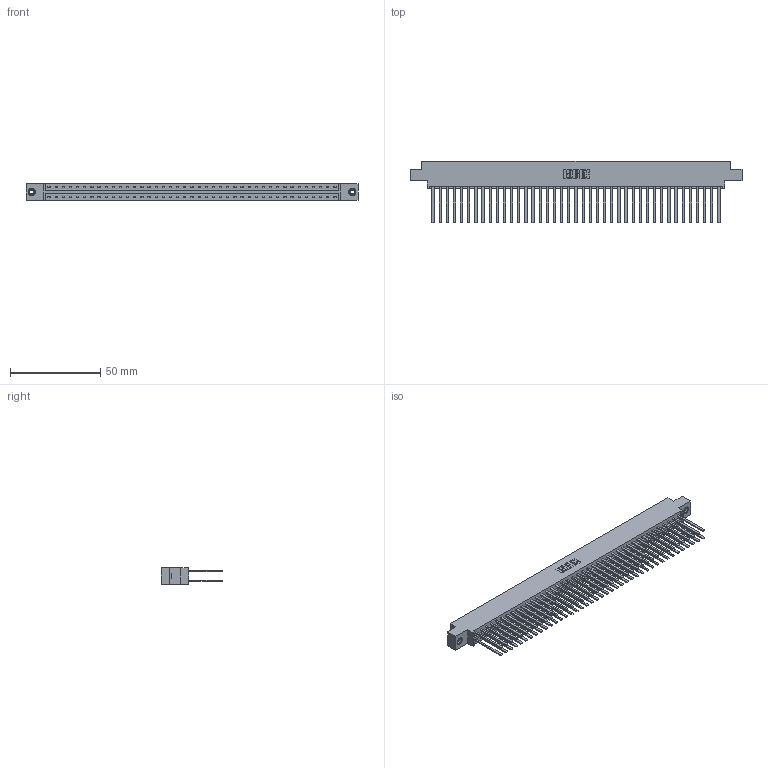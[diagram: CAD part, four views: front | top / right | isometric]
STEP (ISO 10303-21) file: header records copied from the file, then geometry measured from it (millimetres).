
FILE_DESCRIPTION (( 'STEP AP203' ), '1' );
FILE_NAME ('833-082-544-808.STEP', '2020-06-06T00:00:43', ( '' ), ( '' ), 'SwSTEP 2.0', 'SolidWorks 2020', '' );
FILE_SCHEMA (( 'CONFIG_CONTROL_DESIGN' ));
Length unit declared in the file: inch
Products named in the file (4): 833 Part_Offset - .156 Dia - TI; 345-292-001_345-293-144; 345-250-001_345-250-003-102; 833-082-544-808
Assembly tree (85 placements, depth 2):
  833-082-544-808
    833 Part_Offset - .156 Dia - TI
    345-292-001_345-293-144  x82
    345-250-001_345-250-003-102  x2
Bounding box: 184 x 34.3 x 9.4 mm (x, y, z)
Volume: 19690.9 mm3; surface area: 27212.5 mm2
Topology: 85 solids, 85 shells, 3950 faces, 11693 edges, 7678 vertices
Faces by surface type: plane 2730, cylinder 1204, cone 12, torus 4
Entity records: 27640 total; most frequent: CARTESIAN_POINT 4565, ORIENTED_EDGE 4494, DIRECTION 3929, EDGE_CURVE 2247, VECTOR 2103, LINE 2103, VERTEX_POINT 1492, AXIS2_PLACEMENT_3D 913
